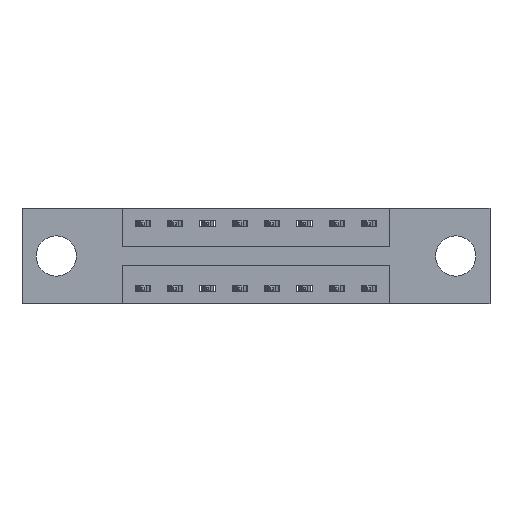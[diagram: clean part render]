
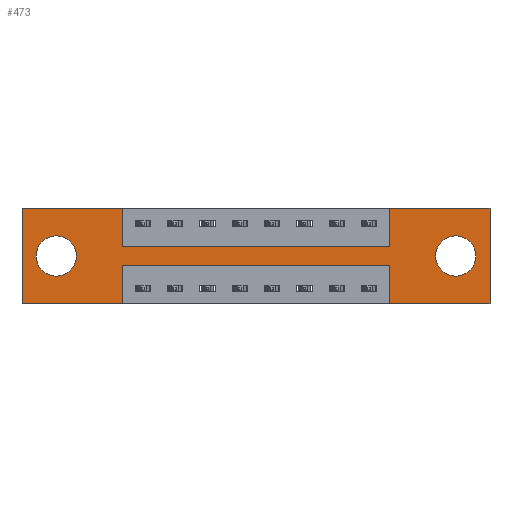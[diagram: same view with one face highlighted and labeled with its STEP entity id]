
A CAD part, front view. The second image highlights one B-rep face of the part: STEP entity #473.
In plain terms, the highlighted planar face has unit normal (0, -1, 0).
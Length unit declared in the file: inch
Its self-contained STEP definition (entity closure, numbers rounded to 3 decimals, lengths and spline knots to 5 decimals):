
#17 = ORIENTED_EDGE ( 'NONE', *, *, #7821, .F. ) ;
#61 = LINE ( 'NONE', #6400, #171 ) ;
#126 = EDGE_LOOP ( 'NONE', ( #5468, #978 ) ) ;
#129 = DIRECTION ( 'NONE',  ( 0., 0., -1. ) ) ;
#171 = VECTOR ( 'NONE', #3400, 39.37008 ) ;
#175 = VERTEX_POINT ( 'NONE', #9734 ) ;
#409 = ORIENTED_EDGE ( 'NONE', *, *, #4266, .T. ) ;
#465 = DIRECTION ( 'NONE',  ( 0., 1., 0. ) ) ;
#473 = ADVANCED_FACE ( 'NONE', ( #2454, #8022, #9579 ), #5075, .T. ) ;
#570 = AXIS2_PLACEMENT_3D ( 'NONE', #1918, #465, #7195 ) ;
#634 = VERTEX_POINT ( 'NONE', #1197 ) ;
#733 = CARTESIAN_POINT ( 'NONE',  ( 0.3875, 0., 0. ) ) ;
#760 = ORIENTED_EDGE ( 'NONE', *, *, #2066, .T. ) ;
#792 = CARTESIAN_POINT ( 'NONE',  ( 1.6775, 0., -0.185 ) ) ;
#836 = CIRCLE ( 'NONE', #6336, 0.078 ) ;
#861 = CARTESIAN_POINT ( 'NONE',  ( 1.6775, 0., -0.263 ) ) ;
#932 = CARTESIAN_POINT ( 'NONE',  ( 0., 0., 0. ) ) ;
#978 = ORIENTED_EDGE ( 'NONE', *, *, #2829, .T. ) ;
#994 = EDGE_CURVE ( 'NONE', #9799, #4587, #3968, .T. ) ;
#1051 = LINE ( 'NONE', #6978, #2901 ) ;
#1167 = VECTOR ( 'NONE', #2318, 39.37008 ) ;
#1197 = CARTESIAN_POINT ( 'NONE',  ( 1.4225, 0., -0.22 ) ) ;
#1295 = VERTEX_POINT ( 'NONE', #7177 ) ;
#1389 = DIRECTION ( 'NONE',  ( 0., 1., 0. ) ) ;
#1410 = CARTESIAN_POINT ( 'NONE',  ( 0., 0., 0. ) ) ;
#1426 = LINE ( 'NONE', #3867, #4823 ) ;
#1583 = ORIENTED_EDGE ( 'NONE', *, *, #4757, .F. ) ;
#1786 = ORIENTED_EDGE ( 'NONE', *, *, #994, .F. ) ;
#1835 = VECTOR ( 'NONE', #3617, 39.37008 ) ;
#1845 = CARTESIAN_POINT ( 'NONE',  ( 1.4225, 0., 0. ) ) ;
#1906 = VECTOR ( 'NONE', #9059, 39.37008 ) ;
#1918 = CARTESIAN_POINT ( 'NONE',  ( 1.6775, 0., -0.185 ) ) ;
#1922 = CIRCLE ( 'NONE', #3008, 0.078 ) ;
#1968 = ORIENTED_EDGE ( 'NONE', *, *, #9128, .F. ) ;
#2065 = LINE ( 'NONE', #8494, #6669 ) ;
#2066 = EDGE_CURVE ( 'NONE', #6847, #8200, #2519, .T. ) ;
#2082 = DIRECTION ( 'NONE',  ( 0., -1., 0. ) ) ;
#2092 = VERTEX_POINT ( 'NONE', #6369 ) ;
#2138 = DIRECTION ( 'NONE',  ( -1., 0., 0. ) ) ;
#2209 = VECTOR ( 'NONE', #7123, 39.37008 ) ;
#2318 = DIRECTION ( 'NONE',  ( 0., 0., 1. ) ) ;
#2440 = DIRECTION ( 'NONE',  ( 0., 0., -1. ) ) ;
#2454 = FACE_BOUND ( 'NONE', #8437, .T. ) ;
#2519 = CIRCLE ( 'NONE', #570, 0.078 ) ;
#2584 = LINE ( 'NONE', #9756, #3027 ) ;
#2620 = VECTOR ( 'NONE', #2138, 39.37008 ) ;
#2747 = EDGE_CURVE ( 'NONE', #634, #3850, #3648, .T. ) ;
#2829 = EDGE_CURVE ( 'NONE', #8652, #5221, #1922, .T. ) ;
#2901 = VECTOR ( 'NONE', #4745, 39.37008 ) ;
#2931 = CARTESIAN_POINT ( 'NONE',  ( 0.3875, 0., 0. ) ) ;
#2975 = CARTESIAN_POINT ( 'NONE',  ( 1.4225, 0., -0.37 ) ) ;
#3008 = AXIS2_PLACEMENT_3D ( 'NONE', #7906, #8779, #5029 ) ;
#3027 = VECTOR ( 'NONE', #5073, 39.37008 ) ;
#3160 = VERTEX_POINT ( 'NONE', #733 ) ;
#3163 = LINE ( 'NONE', #2931, #1906 ) ;
#3275 = ORIENTED_EDGE ( 'NONE', *, *, #3801, .F. ) ;
#3396 = ORIENTED_EDGE ( 'NONE', *, *, #8098, .F. ) ;
#3400 = DIRECTION ( 'NONE',  ( -1., 0., 0. ) ) ;
#3506 = LINE ( 'NONE', #6363, #5055 ) ;
#3617 = DIRECTION ( 'NONE',  ( 0., 0., 1. ) ) ;
#3648 = LINE ( 'NONE', #6733, #2620 ) ;
#3801 = EDGE_CURVE ( 'NONE', #3160, #9089, #3163, .T. ) ;
#3845 = CARTESIAN_POINT ( 'NONE',  ( 0.3875, 0., -0.22 ) ) ;
#3848 = CARTESIAN_POINT ( 'NONE',  ( 1.4225, 0., 0. ) ) ;
#3850 = VERTEX_POINT ( 'NONE', #3845 ) ;
#3867 = CARTESIAN_POINT ( 'NONE',  ( 0.3875, 0., -0.37 ) ) ;
#3890 = DIRECTION ( 'NONE',  ( 1., 0., 0. ) ) ;
#3968 = LINE ( 'NONE', #932, #2209 ) ;
#4229 = CARTESIAN_POINT ( 'NONE',  ( 1.6775, 0., -0.107 ) ) ;
#4266 = EDGE_CURVE ( 'NONE', #8200, #6847, #836, .T. ) ;
#4286 = CARTESIAN_POINT ( 'NONE',  ( 1.81, 0., 0. ) ) ;
#4369 = EDGE_CURVE ( 'NONE', #3850, #1295, #1426, .T. ) ;
#4396 = ORIENTED_EDGE ( 'NONE', *, *, #4369, .F. ) ;
#4453 = EDGE_CURVE ( 'NONE', #9256, #634, #3506, .T. ) ;
#4534 = DIRECTION ( 'NONE',  ( 0., 1., 0. ) ) ;
#4587 = VERTEX_POINT ( 'NONE', #4286 ) ;
#4745 = DIRECTION ( 'NONE',  ( 1., 0., 0. ) ) ;
#4757 = EDGE_CURVE ( 'NONE', #1295, #175, #2584, .T. ) ;
#4823 = VECTOR ( 'NONE', #129, 39.37008 ) ;
#5029 = DIRECTION ( 'NONE',  ( 0., 0., 1. ) ) ;
#5055 = VECTOR ( 'NONE', #7122, 39.37008 ) ;
#5071 = VERTEX_POINT ( 'NONE', #5632 ) ;
#5073 = DIRECTION ( 'NONE',  ( -1., 0., 0. ) ) ;
#5075 = PLANE ( 'NONE',  #7577 ) ;
#5162 = DIRECTION ( 'NONE',  ( 0., 0., 1. ) ) ;
#5221 = VERTEX_POINT ( 'NONE', #7287 ) ;
#5298 = CARTESIAN_POINT ( 'NONE',  ( 0.1325, 0., -0.263 ) ) ;
#5468 = ORIENTED_EDGE ( 'NONE', *, *, #7274, .T. ) ;
#5583 = EDGE_CURVE ( 'NONE', #9089, #2092, #7173, .T. ) ;
#5632 = CARTESIAN_POINT ( 'NONE',  ( 1.81, 0., -0.37 ) ) ;
#5913 = ORIENTED_EDGE ( 'NONE', *, *, #5583, .F. ) ;
#6057 = DIRECTION ( 'NONE',  ( 0., 0., -1. ) ) ;
#6301 = EDGE_LOOP ( 'NONE', ( #4396, #8704, #7576, #3396, #8603, #1786, #9810, #5913, #3275, #1968, #17, #1583 ) ) ;
#6336 = AXIS2_PLACEMENT_3D ( 'NONE', #792, #4534, #6057 ) ;
#6363 = CARTESIAN_POINT ( 'NONE',  ( 1.4225, 0., -0.37 ) ) ;
#6369 = CARTESIAN_POINT ( 'NONE',  ( 1.4225, 0., -0.15 ) ) ;
#6400 = CARTESIAN_POINT ( 'NONE',  ( 0., 0., -0.37 ) ) ;
#6597 = CARTESIAN_POINT ( 'NONE',  ( 0., 0., -0.37 ) ) ;
#6669 = VECTOR ( 'NONE', #2440, 39.37008 ) ;
#6733 = CARTESIAN_POINT ( 'NONE',  ( 0.3875, 0., -0.22 ) ) ;
#6847 = VERTEX_POINT ( 'NONE', #861 ) ;
#6939 = EDGE_CURVE ( 'NONE', #4587, #5071, #2065, .T. ) ;
#6978 = CARTESIAN_POINT ( 'NONE',  ( 0., 0., 0. ) ) ;
#7020 = CIRCLE ( 'NONE', #7427, 0.078 ) ;
#7023 = LINE ( 'NONE', #1410, #1835 ) ;
#7122 = DIRECTION ( 'NONE',  ( 0., 0., 1. ) ) ;
#7123 = DIRECTION ( 'NONE',  ( 1., 0., 0. ) ) ;
#7173 = LINE ( 'NONE', #9716, #9460 ) ;
#7177 = CARTESIAN_POINT ( 'NONE',  ( 0.3875, 0., -0.37 ) ) ;
#7195 = DIRECTION ( 'NONE',  ( 0., 0., -1. ) ) ;
#7274 = EDGE_CURVE ( 'NONE', #5221, #8652, #7020, .T. ) ;
#7287 = CARTESIAN_POINT ( 'NONE',  ( 0.1325, 0., -0.107 ) ) ;
#7359 = DIRECTION ( 'NONE',  ( 0., 0., -1. ) ) ;
#7427 = AXIS2_PLACEMENT_3D ( 'NONE', #9745, #1389, #5162 ) ;
#7576 = ORIENTED_EDGE ( 'NONE', *, *, #4453, .F. ) ;
#7577 = AXIS2_PLACEMENT_3D ( 'NONE', #6597, #2082, #7359 ) ;
#7821 = EDGE_CURVE ( 'NONE', #175, #9777, #7023, .T. ) ;
#7906 = CARTESIAN_POINT ( 'NONE',  ( 0.1325, 0., -0.185 ) ) ;
#7917 = LINE ( 'NONE', #3848, #1167 ) ;
#8022 = FACE_BOUND ( 'NONE', #126, .T. ) ;
#8098 = EDGE_CURVE ( 'NONE', #5071, #9256, #61, .T. ) ;
#8200 = VERTEX_POINT ( 'NONE', #4229 ) ;
#8437 = EDGE_LOOP ( 'NONE', ( #409, #760 ) ) ;
#8494 = CARTESIAN_POINT ( 'NONE',  ( 1.81, 0., 0. ) ) ;
#8603 = ORIENTED_EDGE ( 'NONE', *, *, #6939, .F. ) ;
#8652 = VERTEX_POINT ( 'NONE', #5298 ) ;
#8704 = ORIENTED_EDGE ( 'NONE', *, *, #2747, .F. ) ;
#8779 = DIRECTION ( 'NONE',  ( 0., 1., 0. ) ) ;
#8962 = EDGE_CURVE ( 'NONE', #2092, #9799, #7917, .T. ) ;
#9059 = DIRECTION ( 'NONE',  ( 0., 0., -1. ) ) ;
#9089 = VERTEX_POINT ( 'NONE', #9270 ) ;
#9128 = EDGE_CURVE ( 'NONE', #9777, #3160, #1051, .T. ) ;
#9256 = VERTEX_POINT ( 'NONE', #2975 ) ;
#9270 = CARTESIAN_POINT ( 'NONE',  ( 0.3875, 0., -0.15 ) ) ;
#9400 = CARTESIAN_POINT ( 'NONE',  ( 0., 0., 0. ) ) ;
#9460 = VECTOR ( 'NONE', #3890, 39.37008 ) ;
#9579 = FACE_OUTER_BOUND ( 'NONE', #6301, .T. ) ;
#9716 = CARTESIAN_POINT ( 'NONE',  ( 0.3875, 0., -0.15 ) ) ;
#9734 = CARTESIAN_POINT ( 'NONE',  ( 0., 0., -0.37 ) ) ;
#9745 = CARTESIAN_POINT ( 'NONE',  ( 0.1325, 0., -0.185 ) ) ;
#9756 = CARTESIAN_POINT ( 'NONE',  ( 0., 0., -0.37 ) ) ;
#9777 = VERTEX_POINT ( 'NONE', #9400 ) ;
#9799 = VERTEX_POINT ( 'NONE', #1845 ) ;
#9810 = ORIENTED_EDGE ( 'NONE', *, *, #8962, .F. ) ;
